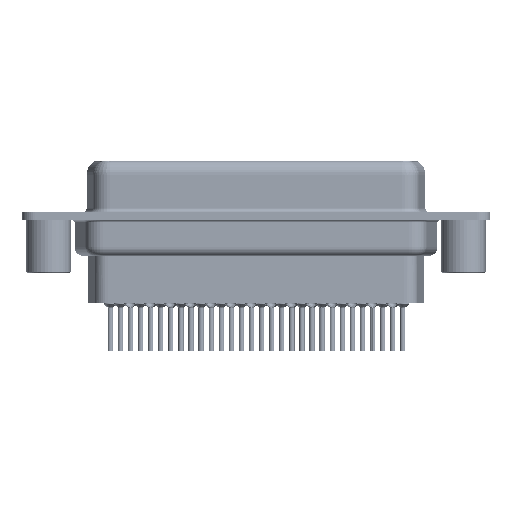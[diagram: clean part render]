
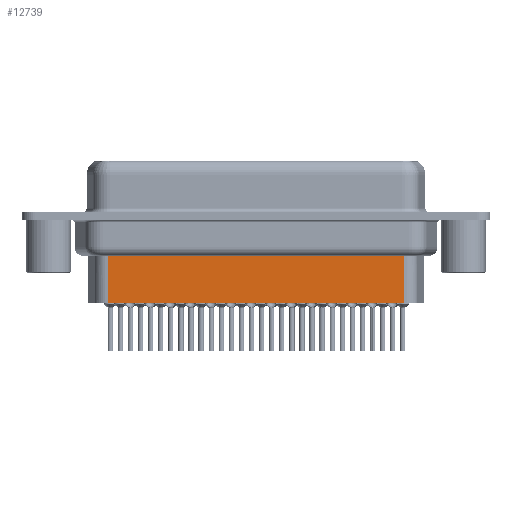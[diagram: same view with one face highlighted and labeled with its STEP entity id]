
A CAD part, front view. The second image highlights one B-rep face of the part: STEP entity #12739.
In plain terms, the highlighted planar face has unit normal (0, -1, 0).
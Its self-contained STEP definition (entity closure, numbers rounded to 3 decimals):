
#71 = AXIS2_PLACEMENT_3D ( 'NONE', #2458, #31316, #12693 ) ;
#439 = VERTEX_POINT ( 'NONE', #14384 ) ;
#685 = EDGE_CURVE ( 'NONE', #27433, #439, #3933, .T. ) ;
#758 = DIRECTION ( 'NONE',  ( -1., 0., 0. ) ) ;
#2134 = CARTESIAN_POINT ( 'NONE',  ( 40.339, -3.5, -4.097 ) ) ;
#2223 = CARTESIAN_POINT ( 'NONE',  ( 40.339, -3.5, -9.85 ) ) ;
#2458 = CARTESIAN_POINT ( 'NONE',  ( 6.701, -3.5, -3.1 ) ) ;
#3524 = CARTESIAN_POINT ( 'NONE',  ( 6.701, -3.5, -9.85 ) ) ;
#3933 = LINE ( 'NONE', #3524, #16847 ) ;
#4157 = VECTOR ( 'NONE', #37452, 1000. ) ;
#4315 = CARTESIAN_POINT ( 'NONE',  ( 6.701, -3.5, -4.097 ) ) ;
#5444 = VECTOR ( 'NONE', #758, 1000. ) ;
#6065 = EDGE_LOOP ( 'NONE', ( #28301, #8272, #25127, #16332 ) ) ;
#6258 = EDGE_CURVE ( 'NONE', #33722, #20551, #34522, .T. ) ;
#6379 = DIRECTION ( 'NONE',  ( -1., 0., 0. ) ) ;
#8272 = ORIENTED_EDGE ( 'NONE', *, *, #6258, .T. ) ;
#11609 = LINE ( 'NONE', #20810, #31356 ) ;
#12235 = DIRECTION ( 'NONE',  ( 0., 0., -1. ) ) ;
#12693 = DIRECTION ( 'NONE',  ( 1., 0., 0. ) ) ;
#12739 = ADVANCED_FACE ( 'NONE', ( #25158 ), #27425, .T. ) ;
#14384 = CARTESIAN_POINT ( 'NONE',  ( 6.701, -3.5, -9.85 ) ) ;
#16332 = ORIENTED_EDGE ( 'NONE', *, *, #685, .F. ) ;
#16847 = VECTOR ( 'NONE', #6379, 1000. ) ;
#17397 = EDGE_CURVE ( 'NONE', #20551, #439, #34382, .T. ) ;
#18419 = CARTESIAN_POINT ( 'NONE',  ( 6.701, -3.5, -3.1 ) ) ;
#20551 = VERTEX_POINT ( 'NONE', #4315 ) ;
#20810 = CARTESIAN_POINT ( 'NONE',  ( 40.339, -3.5, -3.1 ) ) ;
#22213 = CARTESIAN_POINT ( 'NONE',  ( 6.454, -3.5, -4.097 ) ) ;
#25127 = ORIENTED_EDGE ( 'NONE', *, *, #17397, .T. ) ;
#25158 = FACE_OUTER_BOUND ( 'NONE', #6065, .T. ) ;
#27425 = PLANE ( 'NONE',  #71 ) ;
#27433 = VERTEX_POINT ( 'NONE', #2223 ) ;
#28301 = ORIENTED_EDGE ( 'NONE', *, *, #29813, .F. ) ;
#29813 = EDGE_CURVE ( 'NONE', #33722, #27433, #11609, .T. ) ;
#31316 = DIRECTION ( 'NONE',  ( 0., -1., 0. ) ) ;
#31356 = VECTOR ( 'NONE', #12235, 1000. ) ;
#33722 = VERTEX_POINT ( 'NONE', #2134 ) ;
#34382 = LINE ( 'NONE', #18419, #4157 ) ;
#34522 = LINE ( 'NONE', #22213, #5444 ) ;
#37452 = DIRECTION ( 'NONE',  ( 0., 0., -1. ) ) ;
